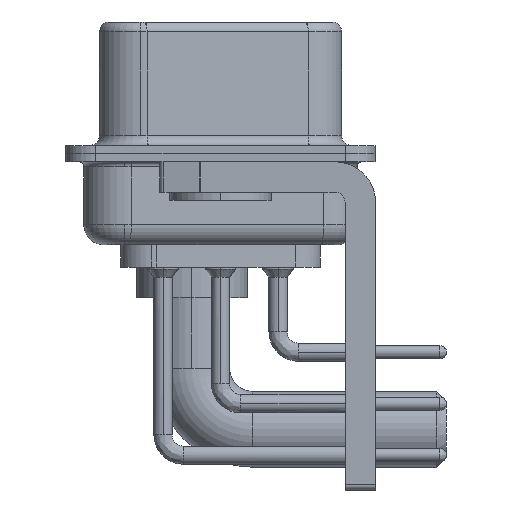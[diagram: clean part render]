
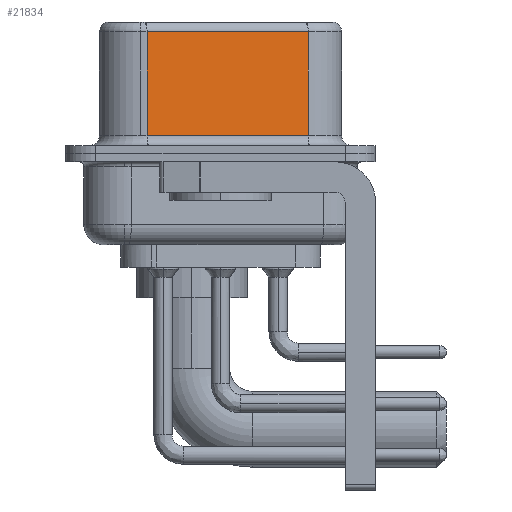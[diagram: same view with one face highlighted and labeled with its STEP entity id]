
A CAD part, left-side view. The second image highlights one B-rep face of the part: STEP entity #21834.
In plain terms, the highlighted planar face has unit normal (-0.985, -0.174, 0).
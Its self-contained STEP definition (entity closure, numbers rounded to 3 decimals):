
#840 = DIRECTION ( 'NONE',  ( 0.985, 0.174, 0. ) ) ;
#1367 = VECTOR ( 'NONE', #30571, 1000. ) ;
#2728 = EDGE_CURVE ( 'NONE', #19867, #13269, #9835, .T. ) ;
#3648 = VERTEX_POINT ( 'NONE', #6759 ) ;
#3845 = FACE_OUTER_BOUND ( 'NONE', #18064, .T. ) ;
#6051 = EDGE_CURVE ( 'NONE', #3648, #9764, #11659, .T. ) ;
#6088 = CARTESIAN_POINT ( 'NONE',  ( 5.132, -4.322, 6.52 ) ) ;
#6759 = CARTESIAN_POINT ( 'NONE',  ( 5.132, -4.322, 6.02 ) ) ;
#8924 = VECTOR ( 'NONE', #29191, 1000. ) ;
#9764 = VERTEX_POINT ( 'NONE', #27325 ) ;
#9835 = LINE ( 'NONE', #27396, #30864 ) ;
#11659 = LINE ( 'NONE', #23071, #23887 ) ;
#13269 = VERTEX_POINT ( 'NONE', #29439 ) ;
#13375 = ORIENTED_EDGE ( 'NONE', *, *, #6051, .F. ) ;
#14677 = DIRECTION ( 'NONE',  ( -0.174, 0.985, 0. ) ) ;
#16319 = LINE ( 'NONE', #33568, #1367 ) ;
#16586 = ORIENTED_EDGE ( 'NONE', *, *, #34917, .T. ) ;
#17743 = CARTESIAN_POINT ( 'NONE',  ( 5.132, -4.322, 0.9 ) ) ;
#18064 = EDGE_LOOP ( 'NONE', ( #13375, #23927, #26505, #16586 ) ) ;
#19802 = EDGE_CURVE ( 'NONE', #3648, #19867, #16319, .T. ) ;
#19867 = VERTEX_POINT ( 'NONE', #25486 ) ;
#20256 = DIRECTION ( 'NONE',  ( 0., 0., -1. ) ) ;
#20572 = LINE ( 'NONE', #17743, #8924 ) ;
#21746 = AXIS2_PLACEMENT_3D ( 'NONE', #6088, #840, #14677 ) ;
#21834 = ADVANCED_FACE ( 'NONE', ( #3845 ), #25912, .F. ) ;
#23071 = CARTESIAN_POINT ( 'NONE',  ( 5.132, -4.322, 6.52 ) ) ;
#23887 = VECTOR ( 'NONE', #20256, 1000. ) ;
#23927 = ORIENTED_EDGE ( 'NONE', *, *, #19802, .T. ) ;
#25486 = CARTESIAN_POINT ( 'NONE',  ( 3.73, 3.628, 6.02 ) ) ;
#25912 = PLANE ( 'NONE',  #21746 ) ;
#26505 = ORIENTED_EDGE ( 'NONE', *, *, #2728, .T. ) ;
#27325 = CARTESIAN_POINT ( 'NONE',  ( 5.132, -4.322, 0.9 ) ) ;
#27396 = CARTESIAN_POINT ( 'NONE',  ( 3.73, 3.628, 6.52 ) ) ;
#29191 = DIRECTION ( 'NONE',  ( 0.174, -0.985, 0. ) ) ;
#29439 = CARTESIAN_POINT ( 'NONE',  ( 3.73, 3.628, 0.9 ) ) ;
#30040 = DIRECTION ( 'NONE',  ( 0., 0., -1. ) ) ;
#30571 = DIRECTION ( 'NONE',  ( -0.174, 0.985, 0. ) ) ;
#30864 = VECTOR ( 'NONE', #30040, 1000. ) ;
#33568 = CARTESIAN_POINT ( 'NONE',  ( 5.132, -4.322, 6.02 ) ) ;
#34917 = EDGE_CURVE ( 'NONE', #13269, #9764, #20572, .T. ) ;
